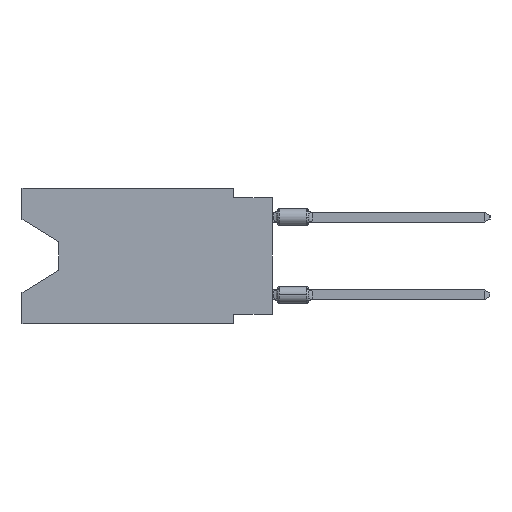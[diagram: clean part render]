
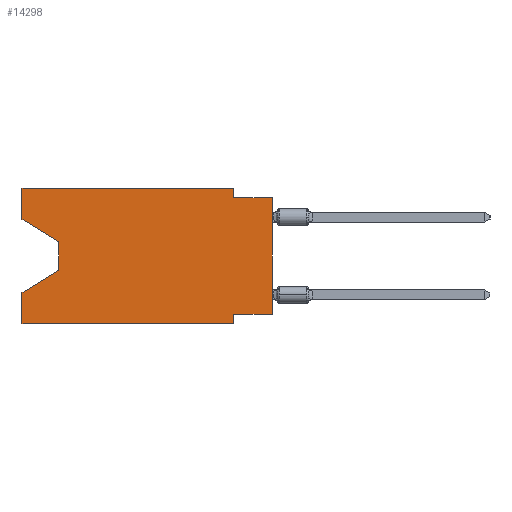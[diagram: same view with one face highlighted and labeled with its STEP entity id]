
A CAD part, left-side view. The second image highlights one B-rep face of the part: STEP entity #14298.
In plain terms, the highlighted planar face has unit normal (-1, 0, 0).
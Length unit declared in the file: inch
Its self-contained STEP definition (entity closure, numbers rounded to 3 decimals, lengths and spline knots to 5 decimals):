
#89 = ORIENTED_EDGE ( 'NONE', *, *, #3591, .F. ) ;
#1072 = VERTEX_POINT ( 'NONE', #45354 ) ;
#1241 = DIRECTION ( 'NONE',  ( 0., -1., 0. ) ) ;
#1348 = EDGE_CURVE ( 'NONE', #26797, #30554, #28083, .T. ) ;
#2243 = VECTOR ( 'NONE', #60640, 39.37008 ) ;
#2387 = ORIENTED_EDGE ( 'NONE', *, *, #53041, .T. ) ;
#2448 = ORIENTED_EDGE ( 'NONE', *, *, #27874, .F. ) ;
#3591 = EDGE_CURVE ( 'NONE', #1072, #30535, #25664, .T. ) ;
#4339 = ORIENTED_EDGE ( 'NONE', *, *, #61100, .T. ) ;
#5505 = CARTESIAN_POINT ( 'NONE',  ( 0., 0., -0.025 ) ) ;
#7469 = ORIENTED_EDGE ( 'NONE', *, *, #59209, .F. ) ;
#8111 = DIRECTION ( 'NONE',  ( 0., 1., 0. ) ) ;
#9091 = CARTESIAN_POINT ( 'NONE',  ( 0., 0., -0.325 ) ) ;
#10230 = DIRECTION ( 'NONE',  ( 0., -0.855, -0.519 ) ) ;
#10715 = LINE ( 'NONE', #39940, #63770 ) ;
#10877 = ORIENTED_EDGE ( 'NONE', *, *, #43102, .F. ) ;
#10956 = VECTOR ( 'NONE', #40294, 39.37008 ) ;
#11056 = EDGE_CURVE ( 'NONE', #28304, #59380, #60011, .T. ) ;
#12179 = VERTEX_POINT ( 'NONE', #29209 ) ;
#12726 = VERTEX_POINT ( 'NONE', #20337 ) ;
#14298 = ADVANCED_FACE ( 'NONE', ( #43021 ), #48534, .F. ) ;
#15383 = VECTOR ( 'NONE', #28442, 39.37008 ) ;
#15706 = CARTESIAN_POINT ( 'NONE',  ( 0., 0.645, -0.35 ) ) ;
#16184 = EDGE_CURVE ( 'NONE', #38007, #26797, #58281, .T. ) ;
#16986 = DIRECTION ( 'NONE',  ( 0., 0., -1. ) ) ;
#17243 = CARTESIAN_POINT ( 'NONE',  ( 0., 0.55, -0.138 ) ) ;
#17487 = DIRECTION ( 'NONE',  ( 0., 0., 1. ) ) ;
#18105 = VECTOR ( 'NONE', #8111, 39.37008 ) ;
#20337 = CARTESIAN_POINT ( 'NONE',  ( 0., 0., -0.325 ) ) ;
#21075 = CARTESIAN_POINT ( 'NONE',  ( 0., 0.645, 0. ) ) ;
#21084 = VECTOR ( 'NONE', #51480, 39.37008 ) ;
#23300 = CARTESIAN_POINT ( 'NONE',  ( 0., 0.1, -0.325 ) ) ;
#23851 = DIRECTION ( 'NONE',  ( 0., 0., -1. ) ) ;
#24703 = ORIENTED_EDGE ( 'NONE', *, *, #16184, .T. ) ;
#25173 = LINE ( 'NONE', #59908, #56768 ) ;
#25664 = LINE ( 'NONE', #60728, #10956 ) ;
#26482 = EDGE_CURVE ( 'NONE', #55130, #59380, #55927, .T. ) ;
#26797 = VERTEX_POINT ( 'NONE', #60087 ) ;
#27874 = EDGE_CURVE ( 'NONE', #12726, #28304, #53573, .T. ) ;
#27896 = CARTESIAN_POINT ( 'NONE',  ( 0., 0.645, -0.35 ) ) ;
#28083 = LINE ( 'NONE', #52429, #21084 ) ;
#28304 = VERTEX_POINT ( 'NONE', #23300 ) ;
#28327 = LINE ( 'NONE', #48141, #38993 ) ;
#28442 = DIRECTION ( 'NONE',  ( 0., 0., 1. ) ) ;
#29068 = VECTOR ( 'NONE', #23851, 39.37008 ) ;
#29209 = CARTESIAN_POINT ( 'NONE',  ( 0., 0.645, -0.08025 ) ) ;
#30460 = CARTESIAN_POINT ( 'NONE',  ( 0., 0.1, -0.35 ) ) ;
#30535 = VERTEX_POINT ( 'NONE', #60316 ) ;
#30554 = VERTEX_POINT ( 'NONE', #35632 ) ;
#30607 = DIRECTION ( 'NONE',  ( 0., -1., 0. ) ) ;
#30792 = LINE ( 'NONE', #5505, #42621 ) ;
#34234 = CARTESIAN_POINT ( 'NONE',  ( 0., 0.55, -0.138 ) ) ;
#35269 = CARTESIAN_POINT ( 'NONE',  ( 0., 0.1, -0.025 ) ) ;
#35632 = CARTESIAN_POINT ( 'NONE',  ( 0., 0.645, -0.26975 ) ) ;
#35992 = DIRECTION ( 'NONE',  ( 0., 0., 1. ) ) ;
#38007 = VERTEX_POINT ( 'NONE', #17243 ) ;
#38993 = VECTOR ( 'NONE', #16986, 39.37008 ) ;
#39940 = CARTESIAN_POINT ( 'NONE',  ( 0., 0., 0. ) ) ;
#40294 = DIRECTION ( 'NONE',  ( 0., -1., 0. ) ) ;
#40770 = VECTOR ( 'NONE', #30607, 39.37008 ) ;
#41411 = ORIENTED_EDGE ( 'NONE', *, *, #48110, .F. ) ;
#42621 = VECTOR ( 'NONE', #1241, 39.37008 ) ;
#43021 = FACE_OUTER_BOUND ( 'NONE', #54781, .T. ) ;
#43102 = EDGE_CURVE ( 'NONE', #12179, #1072, #62849, .T. ) ;
#45354 = CARTESIAN_POINT ( 'NONE',  ( 0., 0.645, 0. ) ) ;
#47250 = VERTEX_POINT ( 'NONE', #35269 ) ;
#47676 = CARTESIAN_POINT ( 'NONE',  ( 0., 0.1, -0.35 ) ) ;
#48110 = EDGE_CURVE ( 'NONE', #47250, #63845, #30792, .T. ) ;
#48141 = CARTESIAN_POINT ( 'NONE',  ( 0., 0.1, 0. ) ) ;
#48534 = PLANE ( 'NONE',  #57047 ) ;
#48906 = CARTESIAN_POINT ( 'NONE',  ( 0., 0.645, 0. ) ) ;
#49704 = ORIENTED_EDGE ( 'NONE', *, *, #57572, .F. ) ;
#51480 = DIRECTION ( 'NONE',  ( 0., 0.855, -0.519 ) ) ;
#52429 = CARTESIAN_POINT ( 'NONE',  ( 0., 0.55, -0.212 ) ) ;
#53041 = EDGE_CURVE ( 'NONE', #12726, #63845, #10715, .T. ) ;
#53395 = CARTESIAN_POINT ( 'NONE',  ( 0., 0.645, 0. ) ) ;
#53573 = LINE ( 'NONE', #9091, #18105 ) ;
#54781 = EDGE_LOOP ( 'NONE', ( #4339, #24703, #59095, #7469, #55060, #62197, #2448, #2387, #41411, #49704, #89, #10877 ) ) ;
#55060 = ORIENTED_EDGE ( 'NONE', *, *, #26482, .T. ) ;
#55130 = VERTEX_POINT ( 'NONE', #27896 ) ;
#55927 = LINE ( 'NONE', #15706, #40770 ) ;
#56768 = VECTOR ( 'NONE', #10230, 39.37008 ) ;
#57047 = AXIS2_PLACEMENT_3D ( 'NONE', #53395, #63778, #62803 ) ;
#57572 = EDGE_CURVE ( 'NONE', #30535, #47250, #28327, .T. ) ;
#58281 = LINE ( 'NONE', #34234, #29068 ) ;
#59095 = ORIENTED_EDGE ( 'NONE', *, *, #1348, .T. ) ;
#59209 = EDGE_CURVE ( 'NONE', #55130, #30554, #61329, .T. ) ;
#59380 = VERTEX_POINT ( 'NONE', #47676 ) ;
#59486 = CARTESIAN_POINT ( 'NONE',  ( 0., 0., -0.025 ) ) ;
#59706 = VECTOR ( 'NONE', #35992, 39.37008 ) ;
#59908 = CARTESIAN_POINT ( 'NONE',  ( 0., 0.645, -0.08025 ) ) ;
#60011 = LINE ( 'NONE', #30460, #2243 ) ;
#60087 = CARTESIAN_POINT ( 'NONE',  ( 0., 0.55, -0.212 ) ) ;
#60316 = CARTESIAN_POINT ( 'NONE',  ( 0., 0.1, 0. ) ) ;
#60640 = DIRECTION ( 'NONE',  ( 0., 0., -1. ) ) ;
#60728 = CARTESIAN_POINT ( 'NONE',  ( 0., 0.645, 0. ) ) ;
#61100 = EDGE_CURVE ( 'NONE', #12179, #38007, #25173, .T. ) ;
#61329 = LINE ( 'NONE', #21075, #59706 ) ;
#62197 = ORIENTED_EDGE ( 'NONE', *, *, #11056, .F. ) ;
#62803 = DIRECTION ( 'NONE',  ( 0., 0., -1. ) ) ;
#62849 = LINE ( 'NONE', #48906, #15383 ) ;
#63770 = VECTOR ( 'NONE', #17487, 39.37008 ) ;
#63778 = DIRECTION ( 'NONE',  ( 1., 0., 0. ) ) ;
#63845 = VERTEX_POINT ( 'NONE', #59486 ) ;
